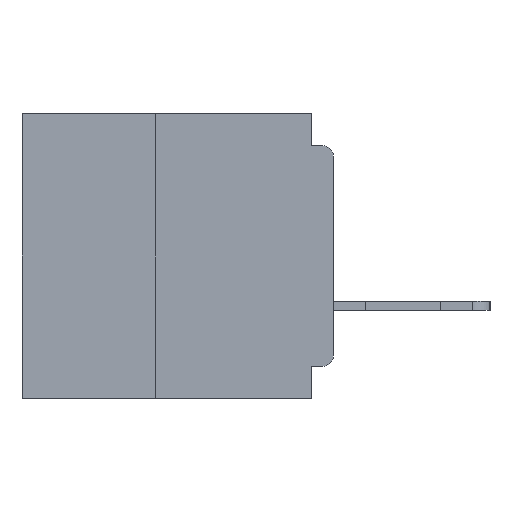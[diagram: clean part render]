
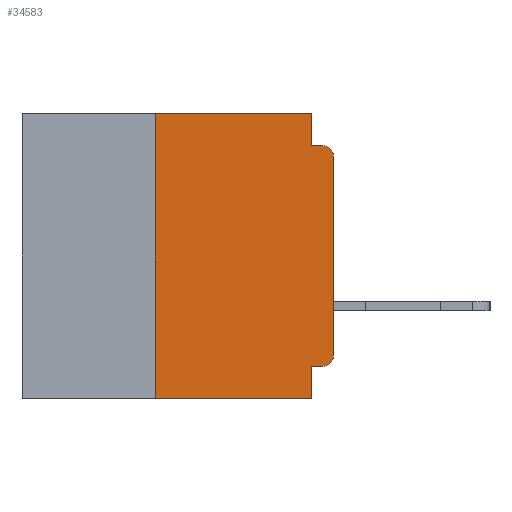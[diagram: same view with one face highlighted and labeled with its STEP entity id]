
A CAD part, left-side view. The second image highlights one B-rep face of the part: STEP entity #34583.
In plain terms, the highlighted planar face has unit normal (-1, 0, 0).
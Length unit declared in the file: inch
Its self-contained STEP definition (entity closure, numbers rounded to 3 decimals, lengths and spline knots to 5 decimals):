
#312 = DIRECTION ( 'NONE',  ( 0., -1., 0. ) ) ;
#1213 = LINE ( 'NONE', #1881, #54647 ) ;
#1758 = FACE_OUTER_BOUND ( 'NONE', #9302, .T. ) ;
#1881 = CARTESIAN_POINT ( 'NONE',  ( 0., 0., 0. ) ) ;
#1966 = CARTESIAN_POINT ( 'NONE',  ( 0., 0., -0.06 ) ) ;
#2253 = EDGE_CURVE ( 'NONE', #52290, #29353, #45440, .T. ) ;
#2631 = EDGE_CURVE ( 'NONE', #23114, #29286, #50653, .T. ) ;
#3403 = DIRECTION ( 'NONE',  ( 0., 1., 0. ) ) ;
#4490 = EDGE_CURVE ( 'NONE', #52290, #16177, #36556, .T. ) ;
#5780 = VECTOR ( 'NONE', #312, 39.37008 ) ;
#6048 = CARTESIAN_POINT ( 'NONE',  ( 0., 0., -0.355 ) ) ;
#6114 = DIRECTION ( 'NONE',  ( 0., 0., 1. ) ) ;
#6807 = VERTEX_POINT ( 'NONE', #24149 ) ;
#9074 = EDGE_CURVE ( 'NONE', #10174, #23114, #28678, .T. ) ;
#9302 = EDGE_LOOP ( 'NONE', ( #50635, #24603, #53194, #10890, #18408, #44562, #28631, #20928, #10952, #28493 ) ) ;
#9791 = EDGE_CURVE ( 'NONE', #6807, #10174, #31231, .T. ) ;
#10021 = VERTEX_POINT ( 'NONE', #28221 ) ;
#10174 = VERTEX_POINT ( 'NONE', #12533 ) ;
#10692 = CARTESIAN_POINT ( 'NONE',  ( 0., 0.031, -0.045 ) ) ;
#10873 = CARTESIAN_POINT ( 'NONE',  ( 0., 0.031, -0.355 ) ) ;
#10890 = ORIENTED_EDGE ( 'NONE', *, *, #2631, .F. ) ;
#10928 = EDGE_CURVE ( 'NONE', #32684, #14140, #38459, .T. ) ;
#10952 = ORIENTED_EDGE ( 'NONE', *, *, #2253, .F. ) ;
#11379 = EDGE_CURVE ( 'NONE', #29353, #10021, #39735, .T. ) ;
#11521 = CARTESIAN_POINT ( 'NONE',  ( 0., 0.437, 0. ) ) ;
#12533 = CARTESIAN_POINT ( 'NONE',  ( 0., 0.25, 0. ) ) ;
#14121 = DIRECTION ( 'NONE',  ( -1., 0., 0. ) ) ;
#14140 = VERTEX_POINT ( 'NONE', #42449 ) ;
#15756 = DIRECTION ( 'NONE',  ( 0., 0., -1. ) ) ;
#16177 = VERTEX_POINT ( 'NONE', #44335 ) ;
#16316 = CARTESIAN_POINT ( 'NONE',  ( 0., 0.015, -0.355 ) ) ;
#18408 = ORIENTED_EDGE ( 'NONE', *, *, #9074, .F. ) ;
#19976 = VECTOR ( 'NONE', #41161, 39.37008 ) ;
#20928 = ORIENTED_EDGE ( 'NONE', *, *, #11379, .F. ) ;
#21119 = EDGE_CURVE ( 'NONE', #6807, #10021, #39435, .T. ) ;
#21802 = EDGE_CURVE ( 'NONE', #29286, #14140, #37368, .T. ) ;
#23114 = VERTEX_POINT ( 'NONE', #29761 ) ;
#24149 = CARTESIAN_POINT ( 'NONE',  ( 0., 0.25, -0.4 ) ) ;
#24603 = ORIENTED_EDGE ( 'NONE', *, *, #10928, .T. ) ;
#25312 = DIRECTION ( 'NONE',  ( 0., 0., -1. ) ) ;
#25350 = CARTESIAN_POINT ( 'NONE',  ( 0., 0.437, -0.4 ) ) ;
#28221 = CARTESIAN_POINT ( 'NONE',  ( 0., 0.031, -0.4 ) ) ;
#28482 = VECTOR ( 'NONE', #25312, 39.37008 ) ;
#28493 = ORIENTED_EDGE ( 'NONE', *, *, #4490, .T. ) ;
#28631 = ORIENTED_EDGE ( 'NONE', *, *, #21119, .T. ) ;
#28678 = LINE ( 'NONE', #35891, #48534 ) ;
#29286 = VERTEX_POINT ( 'NONE', #10692 ) ;
#29353 = VERTEX_POINT ( 'NONE', #10873 ) ;
#29761 = CARTESIAN_POINT ( 'NONE',  ( 0., 0.031, 0. ) ) ;
#31231 = LINE ( 'NONE', #32676, #19976 ) ;
#32482 = DIRECTION ( 'NONE',  ( 0., -1., 0. ) ) ;
#32542 = PLANE ( 'NONE',  #41167 ) ;
#32676 = CARTESIAN_POINT ( 'NONE',  ( 0., 0.25, -0.4 ) ) ;
#32684 = VERTEX_POINT ( 'NONE', #1966 ) ;
#33979 = DIRECTION ( 'NONE',  ( 0., 0., -1. ) ) ;
#33997 = DIRECTION ( 'NONE',  ( -1., 0., 0. ) ) ;
#34044 = CARTESIAN_POINT ( 'NONE',  ( 0., 0.015, -0.34 ) ) ;
#34162 = VECTOR ( 'NONE', #3403, 39.37008 ) ;
#34583 = ADVANCED_FACE ( 'NONE', ( #1758 ), #32542, .F. ) ;
#35891 = CARTESIAN_POINT ( 'NONE',  ( 0., 0.437, 0. ) ) ;
#36038 = VECTOR ( 'NONE', #32482, 39.37008 ) ;
#36556 = CIRCLE ( 'NONE', #45683, 0.015 ) ;
#37368 = LINE ( 'NONE', #40971, #36038 ) ;
#38459 = CIRCLE ( 'NONE', #50505, 0.015 ) ;
#39425 = VECTOR ( 'NONE', #49214, 39.37008 ) ;
#39429 = CARTESIAN_POINT ( 'NONE',  ( 0., 0.015, -0.06 ) ) ;
#39435 = LINE ( 'NONE', #25350, #5780 ) ;
#39735 = LINE ( 'NONE', #42170, #28482 ) ;
#40971 = CARTESIAN_POINT ( 'NONE',  ( 0., 0., -0.045 ) ) ;
#41041 = DIRECTION ( 'NONE',  ( 1., 0., 0. ) ) ;
#41161 = DIRECTION ( 'NONE',  ( 0., 0., 1. ) ) ;
#41167 = AXIS2_PLACEMENT_3D ( 'NONE', #11521, #41041, #15756 ) ;
#42170 = CARTESIAN_POINT ( 'NONE',  ( 0., 0.031, -0.4 ) ) ;
#42449 = CARTESIAN_POINT ( 'NONE',  ( 0., 0.015, -0.045 ) ) ;
#42960 = EDGE_CURVE ( 'NONE', #16177, #32684, #1213, .T. ) ;
#43688 = DIRECTION ( 'NONE',  ( 0., 0., -1. ) ) ;
#44335 = CARTESIAN_POINT ( 'NONE',  ( 0., 0., -0.34 ) ) ;
#44420 = DIRECTION ( 'NONE',  ( 0., -1., 0. ) ) ;
#44562 = ORIENTED_EDGE ( 'NONE', *, *, #9791, .F. ) ;
#45440 = LINE ( 'NONE', #6048, #34162 ) ;
#45683 = AXIS2_PLACEMENT_3D ( 'NONE', #34044, #33997, #33979 ) ;
#48534 = VECTOR ( 'NONE', #44420, 39.37008 ) ;
#49214 = DIRECTION ( 'NONE',  ( 0., 0., -1. ) ) ;
#49813 = CARTESIAN_POINT ( 'NONE',  ( 0., 0.031, 0. ) ) ;
#50505 = AXIS2_PLACEMENT_3D ( 'NONE', #39429, #14121, #43688 ) ;
#50635 = ORIENTED_EDGE ( 'NONE', *, *, #42960, .T. ) ;
#50653 = LINE ( 'NONE', #49813, #39425 ) ;
#52290 = VERTEX_POINT ( 'NONE', #16316 ) ;
#53194 = ORIENTED_EDGE ( 'NONE', *, *, #21802, .F. ) ;
#54647 = VECTOR ( 'NONE', #6114, 39.37008 ) ;
